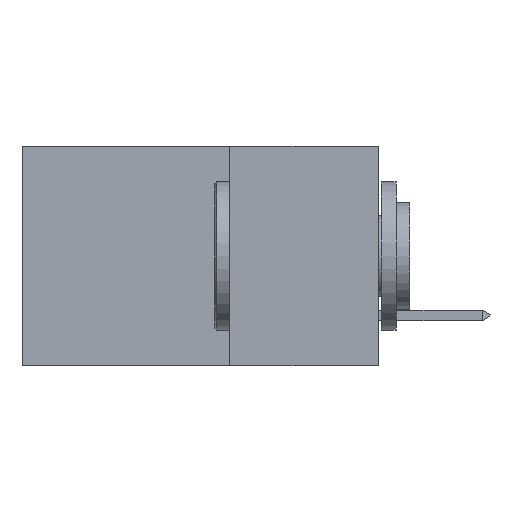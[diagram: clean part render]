
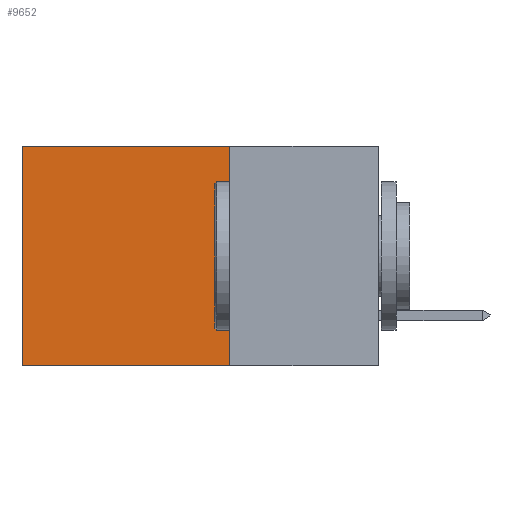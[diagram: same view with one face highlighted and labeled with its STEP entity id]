
A CAD part, left-side view. The second image highlights one B-rep face of the part: STEP entity #9652.
In plain terms, the highlighted planar face has unit normal (-1, 0, 0).
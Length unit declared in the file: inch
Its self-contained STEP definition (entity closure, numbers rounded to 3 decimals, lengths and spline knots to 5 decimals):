
#1210 = VECTOR ( 'NONE', #4941, 39.37008 ) ;
#2774 = AXIS2_PLACEMENT_3D ( 'NONE', #5092, #19538, #12371 ) ;
#2932 = CARTESIAN_POINT ( 'NONE',  ( 0.2615, 0.25, -0.37 ) ) ;
#3035 = CARTESIAN_POINT ( 'NONE',  ( 0.2615, 0.25, -0.37 ) ) ;
#3070 = CARTESIAN_POINT ( 'NONE',  ( 0.2615, 0.25, -0.37 ) ) ;
#4314 = CARTESIAN_POINT ( 'NONE',  ( 0.2615, 0.25, 0. ) ) ;
#4941 = DIRECTION ( 'NONE',  ( 0., 0., -1. ) ) ;
#5092 = CARTESIAN_POINT ( 'NONE',  ( 0.2615, 0.25, -0.37 ) ) ;
#6675 = LINE ( 'NONE', #22684, #13117 ) ;
#7337 = EDGE_CURVE ( 'NONE', #13097, #14306, #13155, .T. ) ;
#8437 = LINE ( 'NONE', #3070, #21473 ) ;
#8564 = CARTESIAN_POINT ( 'NONE',  ( 0.2615, 0.6, 0. ) ) ;
#8841 = EDGE_CURVE ( 'NONE', #17519, #16836, #11996, .T. ) ;
#9652 = ADVANCED_FACE ( 'NONE', ( #21442 ), #12485, .F. ) ;
#11267 = DIRECTION ( 'NONE',  ( 0., 0., -1. ) ) ;
#11348 = EDGE_CURVE ( 'NONE', #17519, #13097, #6675, .T. ) ;
#11802 = EDGE_CURVE ( 'NONE', #16836, #14306, #8437, .T. ) ;
#11996 = LINE ( 'NONE', #3035, #1210 ) ;
#12371 = DIRECTION ( 'NONE',  ( 0., 0., -1. ) ) ;
#12485 = PLANE ( 'NONE',  #2774 ) ;
#13097 = VERTEX_POINT ( 'NONE', #8564 ) ;
#13117 = VECTOR ( 'NONE', #13585, 39.37008 ) ;
#13155 = LINE ( 'NONE', #15163, #21763 ) ;
#13462 = ORIENTED_EDGE ( 'NONE', *, *, #8841, .F. ) ;
#13585 = DIRECTION ( 'NONE',  ( 0., 1., 0. ) ) ;
#14306 = VERTEX_POINT ( 'NONE', #21391 ) ;
#15163 = CARTESIAN_POINT ( 'NONE',  ( 0.2615, 0.6, -0.37 ) ) ;
#15464 = DIRECTION ( 'NONE',  ( 0., 1., 0. ) ) ;
#16222 = ORIENTED_EDGE ( 'NONE', *, *, #7337, .T. ) ;
#16836 = VERTEX_POINT ( 'NONE', #2932 ) ;
#17197 = EDGE_LOOP ( 'NONE', ( #16222, #17995, #13462, #21371 ) ) ;
#17519 = VERTEX_POINT ( 'NONE', #4314 ) ;
#17995 = ORIENTED_EDGE ( 'NONE', *, *, #11802, .F. ) ;
#19538 = DIRECTION ( 'NONE',  ( 1., 0., 0. ) ) ;
#21371 = ORIENTED_EDGE ( 'NONE', *, *, #11348, .T. ) ;
#21391 = CARTESIAN_POINT ( 'NONE',  ( 0.2615, 0.6, -0.37 ) ) ;
#21442 = FACE_OUTER_BOUND ( 'NONE', #17197, .T. ) ;
#21473 = VECTOR ( 'NONE', #15464, 39.37008 ) ;
#21763 = VECTOR ( 'NONE', #11267, 39.37008 ) ;
#22684 = CARTESIAN_POINT ( 'NONE',  ( 0.2615, 0.25, 0. ) ) ;
